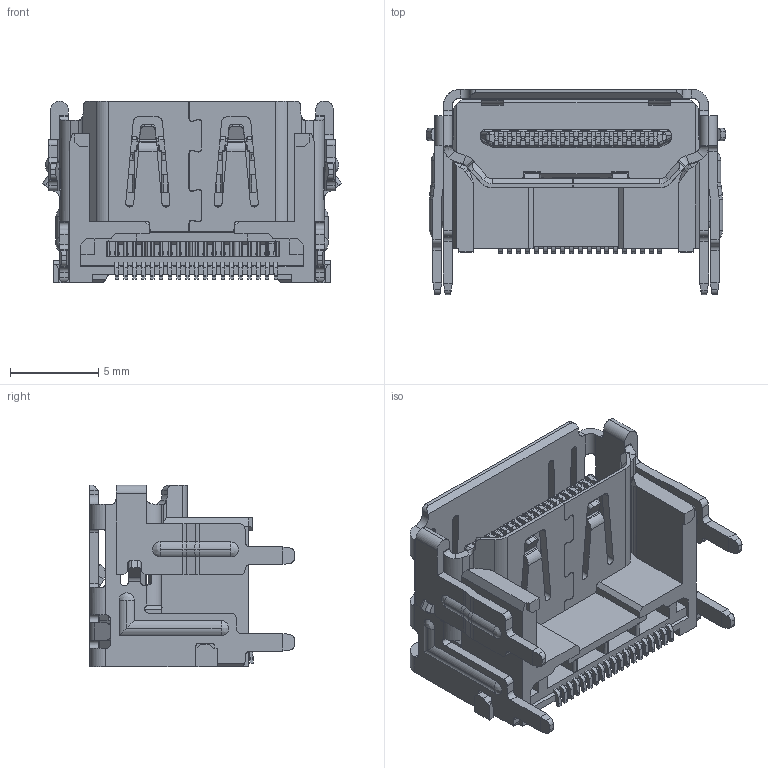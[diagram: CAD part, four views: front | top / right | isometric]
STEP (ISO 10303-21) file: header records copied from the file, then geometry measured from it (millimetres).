
FILE_DESCRIPTION (( 'STEP AP214' ), '1' );
FILE_NAME ('694A619-165-211.STEP', '2021-01-13T13:50:17', ( '' ), ( '' ), 'SwSTEP 2.0', 'SolidWorks 2020', '' );
FILE_SCHEMA (( 'AUTOMOTIVE_DESIGN' ));
Length unit declared in the file: millimetre
Products named in the file (5): Insulator 694A619-X65-211; Contact Lower 694A619-X65-211; Contact Upper 694A619-X65-211; 694A619-165-211; Shell 694A619-X65-211
Assembly tree (21 placements, depth 2):
  694A619-165-211
    Insulator 694A619-X65-211
    Contact Lower 694A619-X65-211  x9
    Contact Upper 694A619-X65-211  x10
    Shell 694A619-X65-211
Bounding box: 16.93 x 11.6 x 10.3 mm (x, y, z)
Volume: 517.7 mm3; surface area: 2096.9 mm2
Topology: 21 solids, 21 shells, 4232 faces, 12236 edges, 7989 vertices
Faces by surface type: plane 2728, cylinder 1379, bspline 110, cone 10, torus 5
Entity records: 100203 total; most frequent: CARTESIAN_POINT 26562, ORIENTED_EDGE 16590, DIRECTION 13531, EDGE_CURVE 8295, VECTOR 5765, LINE 5765, VERTEX_POINT 5371, AXIS2_PLACEMENT_3D 3883
